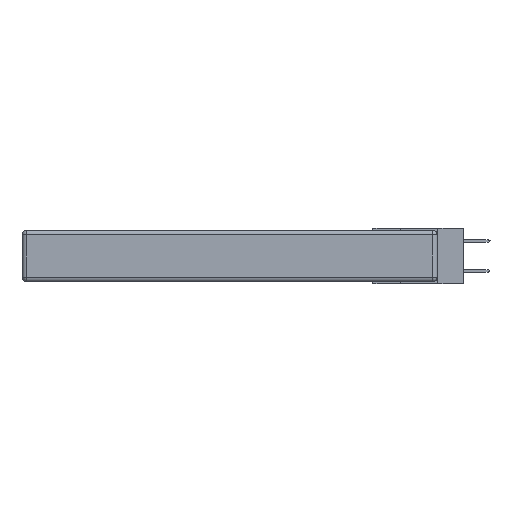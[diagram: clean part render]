
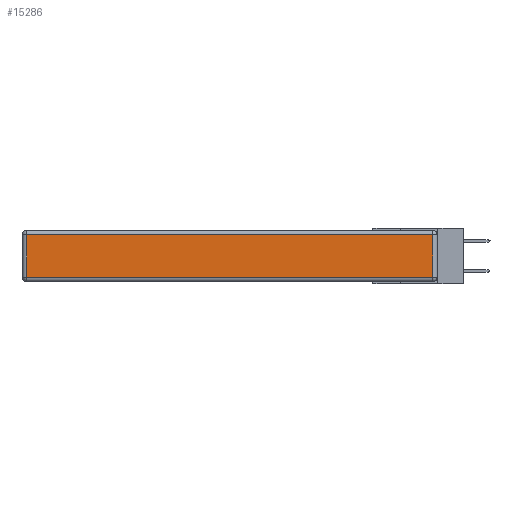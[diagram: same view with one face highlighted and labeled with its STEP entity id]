
A CAD part, left-side view. The second image highlights one B-rep face of the part: STEP entity #15286.
In plain terms, the highlighted planar face has unit normal (-1, 0, 0).
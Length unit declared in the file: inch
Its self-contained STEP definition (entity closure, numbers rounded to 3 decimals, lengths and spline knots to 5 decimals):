
#260 = VERTEX_POINT ( 'NONE', #15010 ) ;
#839 = DIRECTION ( 'NONE',  ( 0., 0., -1. ) ) ;
#2324 = LINE ( 'NONE', #12812, #15658 ) ;
#2540 = ORIENTED_EDGE ( 'NONE', *, *, #16809, .T. ) ;
#5247 = VECTOR ( 'NONE', #20299, 39.37008 ) ;
#6170 = DIRECTION ( 'NONE',  ( 0., 0., 1. ) ) ;
#6180 = CARTESIAN_POINT ( 'NONE',  ( 0., 0., -0.343 ) ) ;
#6685 = VECTOR ( 'NONE', #6819, 39.37008 ) ;
#6819 = DIRECTION ( 'NONE',  ( 0., -1., 0. ) ) ;
#6926 = EDGE_CURVE ( 'NONE', #16283, #12782, #14611, .T. ) ;
#7221 = CARTESIAN_POINT ( 'NONE',  ( 0., 0.03, -0.313 ) ) ;
#9372 = DIRECTION ( 'NONE',  ( 0., 0., 1. ) ) ;
#9518 = DIRECTION ( 'NONE',  ( -1., 0., 0. ) ) ;
#9860 = VECTOR ( 'NONE', #6170, 39.37008 ) ;
#10182 = EDGE_LOOP ( 'NONE', ( #21936, #16914, #2540, #17544 ) ) ;
#11102 = CARTESIAN_POINT ( 'NONE',  ( 0., 0.03, -0.03 ) ) ;
#11192 = AXIS2_PLACEMENT_3D ( 'NONE', #6180, #9518, #9372 ) ;
#11212 = PLANE ( 'NONE',  #11192 ) ;
#11463 = CARTESIAN_POINT ( 'NONE',  ( 0., 2.75, -0.03 ) ) ;
#12782 = VERTEX_POINT ( 'NONE', #7221 ) ;
#12812 = CARTESIAN_POINT ( 'NONE',  ( 0., 2.72, -0.343 ) ) ;
#13143 = VERTEX_POINT ( 'NONE', #11102 ) ;
#13738 = CARTESIAN_POINT ( 'NONE',  ( 0., 0., -0.313 ) ) ;
#14611 = LINE ( 'NONE', #13738, #6685 ) ;
#14838 = CARTESIAN_POINT ( 'NONE',  ( 0., 0.03, -0.343 ) ) ;
#15010 = CARTESIAN_POINT ( 'NONE',  ( 0., 2.72, -0.03 ) ) ;
#15286 = ADVANCED_FACE ( 'NONE', ( #17325 ), #11212, .T. ) ;
#15658 = VECTOR ( 'NONE', #839, 39.37008 ) ;
#16283 = VERTEX_POINT ( 'NONE', #22097 ) ;
#16673 = LINE ( 'NONE', #11463, #5247 ) ;
#16809 = EDGE_CURVE ( 'NONE', #13143, #260, #16673, .T. ) ;
#16914 = ORIENTED_EDGE ( 'NONE', *, *, #20489, .T. ) ;
#17325 = FACE_OUTER_BOUND ( 'NONE', #10182, .T. ) ;
#17544 = ORIENTED_EDGE ( 'NONE', *, *, #18374, .T. ) ;
#18072 = LINE ( 'NONE', #14838, #9860 ) ;
#18374 = EDGE_CURVE ( 'NONE', #260, #16283, #2324, .T. ) ;
#20299 = DIRECTION ( 'NONE',  ( 0., 1., 0. ) ) ;
#20489 = EDGE_CURVE ( 'NONE', #12782, #13143, #18072, .T. ) ;
#21936 = ORIENTED_EDGE ( 'NONE', *, *, #6926, .T. ) ;
#22097 = CARTESIAN_POINT ( 'NONE',  ( 0., 2.72, -0.313 ) ) ;
